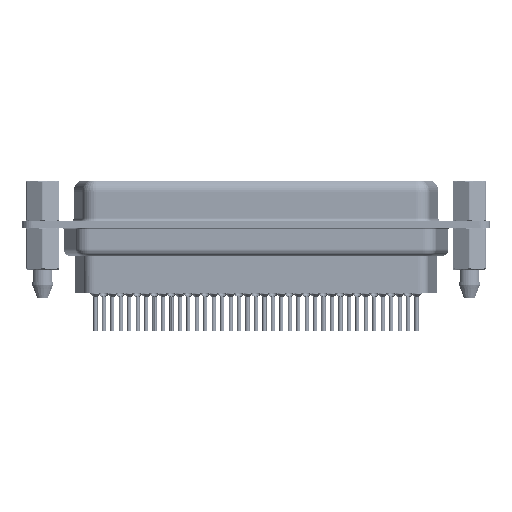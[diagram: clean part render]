
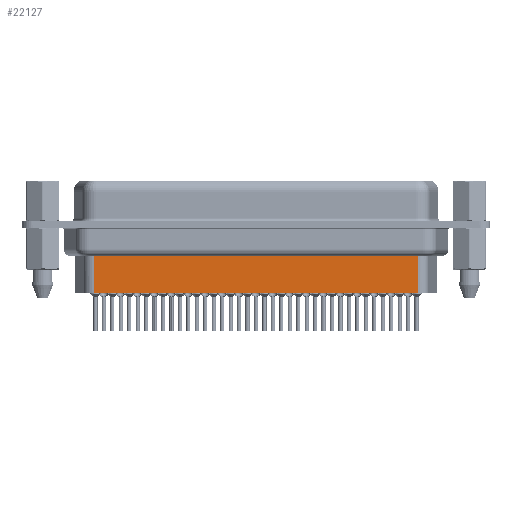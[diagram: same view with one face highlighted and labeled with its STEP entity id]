
A CAD part, front view. The second image highlights one B-rep face of the part: STEP entity #22127.
In plain terms, the highlighted planar face has unit normal (0, -1, 0).
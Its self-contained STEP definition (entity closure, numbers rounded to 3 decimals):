
#7120 = PLANE ( 'NONE',  #11726 ) ;
#7298 = CARTESIAN_POINT ( 'NONE',  ( 53.765, -5., -3.1 ) ) ;
#7628 = DIRECTION ( 'NONE',  ( -1., 0., 0. ) ) ;
#9164 = CARTESIAN_POINT ( 'NONE',  ( 53.765, -5., -4.097 ) ) ;
#11726 = AXIS2_PLACEMENT_3D ( 'NONE', #46026, #21566, #41201 ) ;
#12127 = LINE ( 'NONE', #7298, #42743 ) ;
#14164 = VECTOR ( 'NONE', #15049, 1000. ) ;
#14353 = VECTOR ( 'NONE', #61098, 1000. ) ;
#14474 = VECTOR ( 'NONE', #7628, 1000. ) ;
#15049 = DIRECTION ( 'NONE',  ( 0., 0., -1. ) ) ;
#18254 = CARTESIAN_POINT ( 'NONE',  ( 53.765, -5., -9.85 ) ) ;
#21566 = DIRECTION ( 'NONE',  ( 0., -1., 0. ) ) ;
#22127 = ADVANCED_FACE ( 'NONE', ( #26387 ), #7120, .T. ) ;
#22357 = ORIENTED_EDGE ( 'NONE', *, *, #43252, .T. ) ;
#22724 = CARTESIAN_POINT ( 'NONE',  ( 7.335, -5., -9.85 ) ) ;
#23564 = VERTEX_POINT ( 'NONE', #58423 ) ;
#25179 = VERTEX_POINT ( 'NONE', #9164 ) ;
#26387 = FACE_OUTER_BOUND ( 'NONE', #41753, .T. ) ;
#26897 = DIRECTION ( 'NONE',  ( 0., 0., -1. ) ) ;
#27556 = LINE ( 'NONE', #37840, #14474 ) ;
#31957 = VERTEX_POINT ( 'NONE', #18254 ) ;
#37840 = CARTESIAN_POINT ( 'NONE',  ( 7.335, -5., -9.85 ) ) ;
#40531 = LINE ( 'NONE', #46634, #14353 ) ;
#41201 = DIRECTION ( 'NONE',  ( 1., 0., 0. ) ) ;
#41753 = EDGE_LOOP ( 'NONE', ( #58518, #45511, #22357, #44672 ) ) ;
#41831 = EDGE_CURVE ( 'NONE', #25179, #31957, #12127, .T. ) ;
#42743 = VECTOR ( 'NONE', #26897, 1000. ) ;
#43252 = EDGE_CURVE ( 'NONE', #23564, #57658, #58788, .T. ) ;
#44672 = ORIENTED_EDGE ( 'NONE', *, *, #47744, .F. ) ;
#45511 = ORIENTED_EDGE ( 'NONE', *, *, #55542, .T. ) ;
#46026 = CARTESIAN_POINT ( 'NONE',  ( 7.335, -5., -3.1 ) ) ;
#46634 = CARTESIAN_POINT ( 'NONE',  ( 7.088, -5., -4.097 ) ) ;
#47744 = EDGE_CURVE ( 'NONE', #31957, #57658, #27556, .T. ) ;
#54587 = CARTESIAN_POINT ( 'NONE',  ( 7.335, -5., -3.1 ) ) ;
#55542 = EDGE_CURVE ( 'NONE', #25179, #23564, #40531, .T. ) ;
#57658 = VERTEX_POINT ( 'NONE', #22724 ) ;
#58423 = CARTESIAN_POINT ( 'NONE',  ( 7.335, -5., -4.097 ) ) ;
#58518 = ORIENTED_EDGE ( 'NONE', *, *, #41831, .F. ) ;
#58788 = LINE ( 'NONE', #54587, #14164 ) ;
#61098 = DIRECTION ( 'NONE',  ( -1., 0., 0. ) ) ;
